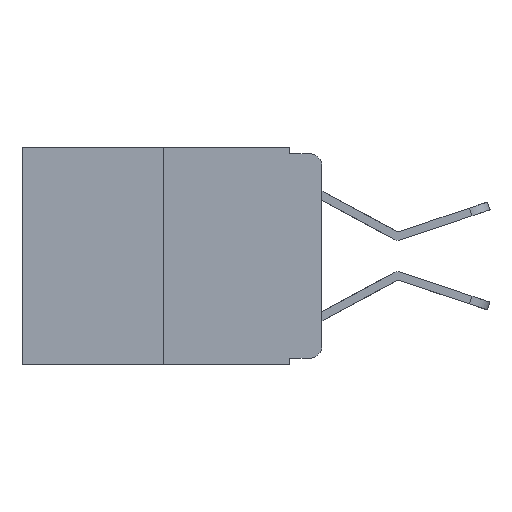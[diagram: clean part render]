
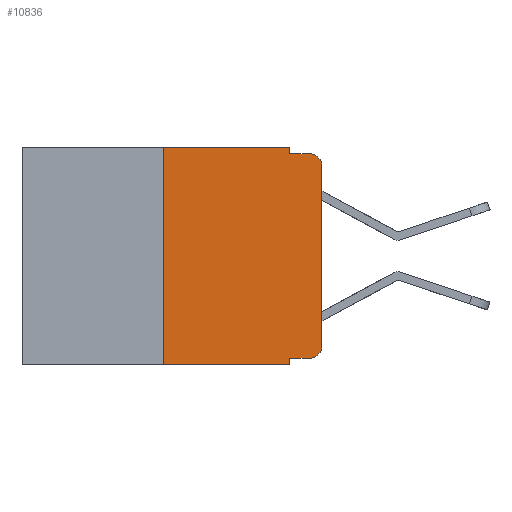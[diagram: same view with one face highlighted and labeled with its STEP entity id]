
A CAD part, left-side view. The second image highlights one B-rep face of the part: STEP entity #10836.
In plain terms, the highlighted planar face has unit normal (-1, 0, 0).
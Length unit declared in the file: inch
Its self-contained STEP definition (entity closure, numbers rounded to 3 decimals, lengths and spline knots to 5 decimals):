
#447 = VECTOR ( 'NONE', #17389, 39.37008 ) ;
#853 = EDGE_CURVE ( 'NONE', #1287, #7964, #12520, .T. ) ;
#1287 = VERTEX_POINT ( 'NONE', #8483 ) ;
#1384 = VECTOR ( 'NONE', #24137, 39.37008 ) ;
#1466 = DIRECTION ( 'NONE',  ( 0., -1., 0. ) ) ;
#2061 = FACE_OUTER_BOUND ( 'NONE', #10451, .T. ) ;
#2243 = CARTESIAN_POINT ( 'NONE',  ( 0., 0.473, -0.343 ) ) ;
#2304 = LINE ( 'NONE', #11155, #21749 ) ;
#2403 = DIRECTION ( 'NONE',  ( 1., 0., 0. ) ) ;
#2957 = LINE ( 'NONE', #7930, #22336 ) ;
#3501 = DIRECTION ( 'NONE',  ( 0., -1., 0. ) ) ;
#3571 = EDGE_CURVE ( 'NONE', #1287, #20289, #10653, .T. ) ;
#3675 = ORIENTED_EDGE ( 'NONE', *, *, #3571, .F. ) ;
#3752 = EDGE_CURVE ( 'NONE', #15756, #7570, #6576, .T. ) ;
#3899 = EDGE_CURVE ( 'NONE', #20289, #18729, #2957, .T. ) ;
#3956 = DIRECTION ( 'NONE',  ( 0., 0., -1. ) ) ;
#4231 = CARTESIAN_POINT ( 'NONE',  ( 0., 0., -0.03 ) ) ;
#4386 = EDGE_CURVE ( 'NONE', #6683, #7964, #2304, .T. ) ;
#4660 = VECTOR ( 'NONE', #3501, 39.37008 ) ;
#5236 = VECTOR ( 'NONE', #24037, 39.37008 ) ;
#5773 = DIRECTION ( 'NONE',  ( -1., 0., 0. ) ) ;
#6576 = LINE ( 'NONE', #10178, #1384 ) ;
#6683 = VERTEX_POINT ( 'NONE', #21850 ) ;
#6741 = DIRECTION ( 'NONE',  ( 0., -1., 0. ) ) ;
#7287 = CARTESIAN_POINT ( 'NONE',  ( 0., 0.051, -0.01 ) ) ;
#7537 = ORIENTED_EDGE ( 'NONE', *, *, #22427, .F. ) ;
#7539 = VECTOR ( 'NONE', #1466, 39.37008 ) ;
#7570 = VERTEX_POINT ( 'NONE', #4231 ) ;
#7930 = CARTESIAN_POINT ( 'NONE',  ( 0., 0.473, 0. ) ) ;
#7964 = VERTEX_POINT ( 'NONE', #20303 ) ;
#8483 = CARTESIAN_POINT ( 'NONE',  ( 0., 0.25, -0.343 ) ) ;
#8779 = AXIS2_PLACEMENT_3D ( 'NONE', #11309, #24347, #13234 ) ;
#8852 = CIRCLE ( 'NONE', #21040, 0.02 ) ;
#9004 = ORIENTED_EDGE ( 'NONE', *, *, #3752, .T. ) ;
#10178 = CARTESIAN_POINT ( 'NONE',  ( 0., 0., 0. ) ) ;
#10209 = LINE ( 'NONE', #7287, #5236 ) ;
#10224 = LINE ( 'NONE', #12897, #4660 ) ;
#10307 = CIRCLE ( 'NONE', #8779, 0.02 ) ;
#10451 = EDGE_LOOP ( 'NONE', ( #9004, #20165, #11304, #7537, #23004, #3675, #24138, #10465, #21037, #17231 ) ) ;
#10465 = ORIENTED_EDGE ( 'NONE', *, *, #4386, .F. ) ;
#10653 = LINE ( 'NONE', #14928, #447 ) ;
#10836 = ADVANCED_FACE ( 'NONE', ( #2061 ), #21193, .F. ) ;
#11155 = CARTESIAN_POINT ( 'NONE',  ( 0., 0.051, 0. ) ) ;
#11304 = ORIENTED_EDGE ( 'NONE', *, *, #17309, .F. ) ;
#11309 = CARTESIAN_POINT ( 'NONE',  ( 0., 0.02, -0.313 ) ) ;
#11515 = AXIS2_PLACEMENT_3D ( 'NONE', #23007, #2403, #15636 ) ;
#12520 = LINE ( 'NONE', #2243, #7539 ) ;
#12711 = EDGE_CURVE ( 'NONE', #17469, #15756, #10307, .T. ) ;
#12897 = CARTESIAN_POINT ( 'NONE',  ( 0., 0.051, -0.333 ) ) ;
#13234 = DIRECTION ( 'NONE',  ( 0., 0., -1. ) ) ;
#14644 = EDGE_CURVE ( 'NONE', #7570, #18793, #8852, .T. ) ;
#14928 = CARTESIAN_POINT ( 'NONE',  ( 0., 0.25, 0. ) ) ;
#15147 = CARTESIAN_POINT ( 'NONE',  ( 0., 0.02, -0.333 ) ) ;
#15636 = DIRECTION ( 'NONE',  ( 0., 0., -1. ) ) ;
#15699 = VERTEX_POINT ( 'NONE', #20792 ) ;
#15756 = VERTEX_POINT ( 'NONE', #17266 ) ;
#16175 = EDGE_CURVE ( 'NONE', #6683, #17469, #10224, .T. ) ;
#16929 = CARTESIAN_POINT ( 'NONE',  ( 0., 0.25, 0. ) ) ;
#17001 = CARTESIAN_POINT ( 'NONE',  ( 0., 0.02, -0.03 ) ) ;
#17231 = ORIENTED_EDGE ( 'NONE', *, *, #12711, .T. ) ;
#17266 = CARTESIAN_POINT ( 'NONE',  ( 0., 0., -0.313 ) ) ;
#17309 = EDGE_CURVE ( 'NONE', #15699, #18793, #10209, .T. ) ;
#17389 = DIRECTION ( 'NONE',  ( 0., 0., 1. ) ) ;
#17469 = VERTEX_POINT ( 'NONE', #15147 ) ;
#18479 = CARTESIAN_POINT ( 'NONE',  ( 0., 0.02, -0.01 ) ) ;
#18729 = VERTEX_POINT ( 'NONE', #23764 ) ;
#18793 = VERTEX_POINT ( 'NONE', #18479 ) ;
#18905 = DIRECTION ( 'NONE',  ( 0., 0., -1. ) ) ;
#19460 = VECTOR ( 'NONE', #3956, 39.37008 ) ;
#20165 = ORIENTED_EDGE ( 'NONE', *, *, #14644, .T. ) ;
#20289 = VERTEX_POINT ( 'NONE', #16929 ) ;
#20303 = CARTESIAN_POINT ( 'NONE',  ( 0., 0.051, -0.343 ) ) ;
#20792 = CARTESIAN_POINT ( 'NONE',  ( 0., 0.051, -0.01 ) ) ;
#21037 = ORIENTED_EDGE ( 'NONE', *, *, #16175, .T. ) ;
#21040 = AXIS2_PLACEMENT_3D ( 'NONE', #17001, #5773, #18905 ) ;
#21193 = PLANE ( 'NONE',  #11515 ) ;
#21375 = DIRECTION ( 'NONE',  ( 0., 0., -1. ) ) ;
#21749 = VECTOR ( 'NONE', #21375, 39.37008 ) ;
#21850 = CARTESIAN_POINT ( 'NONE',  ( 0., 0.051, -0.333 ) ) ;
#22336 = VECTOR ( 'NONE', #6741, 39.37008 ) ;
#22427 = EDGE_CURVE ( 'NONE', #18729, #15699, #24298, .T. ) ;
#23004 = ORIENTED_EDGE ( 'NONE', *, *, #3899, .F. ) ;
#23007 = CARTESIAN_POINT ( 'NONE',  ( 0., 0.473, 0. ) ) ;
#23764 = CARTESIAN_POINT ( 'NONE',  ( 0., 0.051, 0. ) ) ;
#24037 = DIRECTION ( 'NONE',  ( 0., -1., 0. ) ) ;
#24137 = DIRECTION ( 'NONE',  ( 0., 0., 1. ) ) ;
#24138 = ORIENTED_EDGE ( 'NONE', *, *, #853, .T. ) ;
#24298 = LINE ( 'NONE', #24427, #19460 ) ;
#24347 = DIRECTION ( 'NONE',  ( -1., 0., 0. ) ) ;
#24427 = CARTESIAN_POINT ( 'NONE',  ( 0., 0.051, 0. ) ) ;
